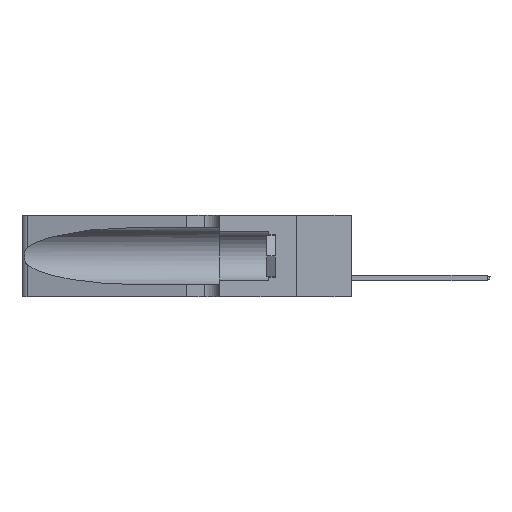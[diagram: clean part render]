
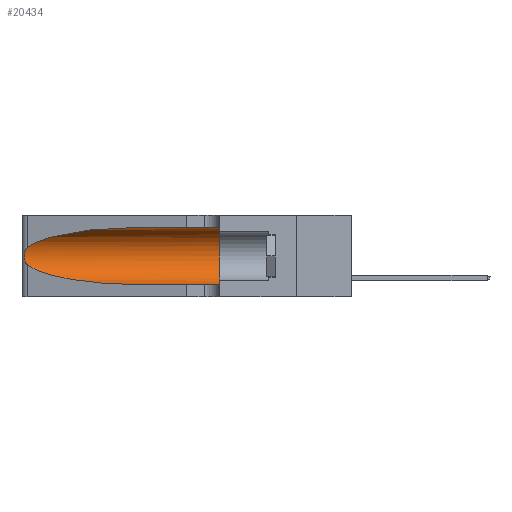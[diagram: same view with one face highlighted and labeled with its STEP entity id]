
A CAD part, left-side view. The second image highlights one B-rep face of the part: STEP entity #20434.
In plain terms, the highlighted cylindrical face has radius 3.308 mm (diameter 6.617 mm), a partial arc.
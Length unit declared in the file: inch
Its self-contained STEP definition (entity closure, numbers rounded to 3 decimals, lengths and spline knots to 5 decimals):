
#658 = EDGE_CURVE ( 'NONE', #15204, #29835, #11101, .T. ) ;
#828 = CARTESIAN_POINT ( 'NONE',  ( 0.1305, 1.61858, 0.185 ) ) ;
#980 = VECTOR ( 'NONE', #22053, 39.37008 ) ;
#2404 = ORIENTED_EDGE ( 'NONE', *, *, #7433, .T. ) ;
#2417 = EDGE_CURVE ( 'NONE', #34567, #15204, #11607, .T. ) ;
#4234 = ORIENTED_EDGE ( 'NONE', *, *, #4494, .F. ) ;
#4494 = EDGE_CURVE ( 'NONE', #26060, #8180, #36205, .T. ) ;
#4800 = CARTESIAN_POINT ( 'NONE',  ( 0.25487, 1.22718, 0.14631 ) ) ;
#6270 = DIRECTION ( 'NONE',  ( 0., 1., 0. ) ) ;
#6378 = CARTESIAN_POINT ( 'NONE',  ( 0.1305, 0.72297, 0.05475 ) ) ;
#6767 = ORIENTED_EDGE ( 'NONE', *, *, #2417, .T. ) ;
#6935 =( BOUNDED_CURVE ( )  B_SPLINE_CURVE ( 3, ( #39236, #23839, #33153, #36273 ),
 .UNSPECIFIED., .F., .F. ) 
 B_SPLINE_CURVE_WITH_KNOTS ( ( 4, 4 ),
 ( 3.44316, 4.71239 ),
 .UNSPECIFIED. ) 
 CURVE ( )  GEOMETRIC_REPRESENTATION_ITEM ( )  RATIONAL_B_SPLINE_CURVE ( ( 1., 0.87, 0.87, 1. ) ) 
 REPRESENTATION_ITEM ( '' )  );
#7173 = DIRECTION ( 'NONE',  ( 0., -1., 0. ) ) ;
#7398 = EDGE_CURVE ( 'NONE', #34567, #26060, #16424, .T. ) ;
#7433 = EDGE_CURVE ( 'NONE', #29835, #34251, #6935, .T. ) ;
#8180 = VERTEX_POINT ( 'NONE', #24850 ) ;
#8594 = CARTESIAN_POINT ( 'NONE',  ( 0.25487, 1.22718, 0.22369 ) ) ;
#8730 = CARTESIAN_POINT ( 'NONE',  ( 0.26018, 1.23835, 0.19895 ) ) ;
#11101 = B_SPLINE_CURVE_WITH_KNOTS ( 'NONE', 3,
 ( #8594, #30151, #18011, #27180, #11934, #8730, #11659, #23941, #15035, #17611, #11804, #27457, #23809, #26915 ),
 .UNSPECIFIED., .F., .F.,
 ( 4, 2, 2, 2, 2, 2, 4 ),
 ( 0., 0.00027, 0.00053, 0.00107, 0.0016, 0.00187, 0.00214 ),
 .UNSPECIFIED. ) ;
#11213 = ORIENTED_EDGE ( 'NONE', *, *, #7398, .F. ) ;
#11607 =( BOUNDED_CURVE ( )  B_SPLINE_CURVE ( 3, ( #12905, #31815, #38147, #25306 ),
 .UNSPECIFIED., .F., .F. ) 
 B_SPLINE_CURVE_WITH_KNOTS ( ( 4, 4 ),
 ( 1.5708, 2.84003 ),
 .UNSPECIFIED. ) 
 CURVE ( )  GEOMETRIC_REPRESENTATION_ITEM ( )  RATIONAL_B_SPLINE_CURVE ( ( 1., 0.87, 0.87, 1. ) ) 
 REPRESENTATION_ITEM ( '' )  );
#11659 = CARTESIAN_POINT ( 'NONE',  ( 0.26075, 1.23896, 0.19203 ) ) ;
#11804 = CARTESIAN_POINT ( 'NONE',  ( 0.25789, 1.23486, 0.15765 ) ) ;
#11934 = CARTESIAN_POINT ( 'NONE',  ( 0.25854, 1.2359, 0.20912 ) ) ;
#12905 = CARTESIAN_POINT ( 'NONE',  ( 0.1305, 0.72297, 0.31525 ) ) ;
#13632 = CARTESIAN_POINT ( 'NONE',  ( 0.1305, 0.35, 0.31525 ) ) ;
#13667 = EDGE_CURVE ( 'NONE', #34251, #8180, #25053, .T. ) ;
#15035 = CARTESIAN_POINT ( 'NONE',  ( 0.26017, 1.23833, 0.17102 ) ) ;
#15204 = VERTEX_POINT ( 'NONE', #38680 ) ;
#16001 = ORIENTED_EDGE ( 'NONE', *, *, #658, .T. ) ;
#16424 = LINE ( 'NONE', #27214, #28508 ) ;
#17495 = DIRECTION ( 'NONE',  ( 0., -1., 0. ) ) ;
#17611 = CARTESIAN_POINT ( 'NONE',  ( 0.25856, 1.23593, 0.16098 ) ) ;
#18011 = CARTESIAN_POINT ( 'NONE',  ( 0.25639, 1.23184, 0.21858 ) ) ;
#18539 = CARTESIAN_POINT ( 'NONE',  ( 0.1305, 0.35, 0.185 ) ) ;
#18975 = EDGE_LOOP ( 'NONE', ( #6767, #16001, #2404, #35727, #4234, #11213 ) ) ;
#20336 = AXIS2_PLACEMENT_3D ( 'NONE', #18539, #6270, #24338 ) ;
#20434 = ADVANCED_FACE ( 'NONE', ( #27633 ), #37777, .F. ) ;
#22053 = DIRECTION ( 'NONE',  ( 0., -1., 0. ) ) ;
#22560 = CARTESIAN_POINT ( 'NONE',  ( 0.1305, 0.72297, 0.31525 ) ) ;
#23809 = CARTESIAN_POINT ( 'NONE',  ( 0.25555, 1.22993, 0.14849 ) ) ;
#23839 = CARTESIAN_POINT ( 'NONE',  ( 0.2373, 1.15595, 0.08982 ) ) ;
#23941 = CARTESIAN_POINT ( 'NONE',  ( 0.26075, 1.23896, 0.178 ) ) ;
#24338 = DIRECTION ( 'NONE',  ( 0., 0., 1. ) ) ;
#24472 = CARTESIAN_POINT ( 'NONE',  ( 0.1305, 1.61858, 0.05475 ) ) ;
#24850 = CARTESIAN_POINT ( 'NONE',  ( 0.1305, 0.35, 0.05475 ) ) ;
#25053 = LINE ( 'NONE', #24472, #980 ) ;
#25306 = CARTESIAN_POINT ( 'NONE',  ( 0.25487, 1.22718, 0.22369 ) ) ;
#26060 = VERTEX_POINT ( 'NONE', #13632 ) ;
#26138 = DIRECTION ( 'NONE',  ( 0., 0., -1. ) ) ;
#26915 = CARTESIAN_POINT ( 'NONE',  ( 0.25487, 1.22718, 0.14631 ) ) ;
#27180 = CARTESIAN_POINT ( 'NONE',  ( 0.25787, 1.23484, 0.2124 ) ) ;
#27214 = CARTESIAN_POINT ( 'NONE',  ( 0.1305, 1.61858, 0.31525 ) ) ;
#27221 = AXIS2_PLACEMENT_3D ( 'NONE', #828, #7173, #26138 ) ;
#27457 = CARTESIAN_POINT ( 'NONE',  ( 0.25639, 1.23186, 0.15144 ) ) ;
#27633 = FACE_OUTER_BOUND ( 'NONE', #18975, .T. ) ;
#28508 = VECTOR ( 'NONE', #17495, 39.37008 ) ;
#29835 = VERTEX_POINT ( 'NONE', #4800 ) ;
#30151 = CARTESIAN_POINT ( 'NONE',  ( 0.25555, 1.22994, 0.2215 ) ) ;
#31815 = CARTESIAN_POINT ( 'NONE',  ( 0.18966, 0.96281, 0.31525 ) ) ;
#33153 = CARTESIAN_POINT ( 'NONE',  ( 0.18966, 0.96281, 0.05475 ) ) ;
#34251 = VERTEX_POINT ( 'NONE', #6378 ) ;
#34567 = VERTEX_POINT ( 'NONE', #22560 ) ;
#35727 = ORIENTED_EDGE ( 'NONE', *, *, #13667, .T. ) ;
#36205 = CIRCLE ( 'NONE', #20336, 0.13025 ) ;
#36273 = CARTESIAN_POINT ( 'NONE',  ( 0.1305, 0.72297, 0.05475 ) ) ;
#37777 = CYLINDRICAL_SURFACE ( 'NONE', #27221, 0.13025 ) ;
#38147 = CARTESIAN_POINT ( 'NONE',  ( 0.2373, 1.15595, 0.28018 ) ) ;
#38680 = CARTESIAN_POINT ( 'NONE',  ( 0.25487, 1.22718, 0.22369 ) ) ;
#39236 = CARTESIAN_POINT ( 'NONE',  ( 0.25487, 1.22718, 0.14631 ) ) ;
